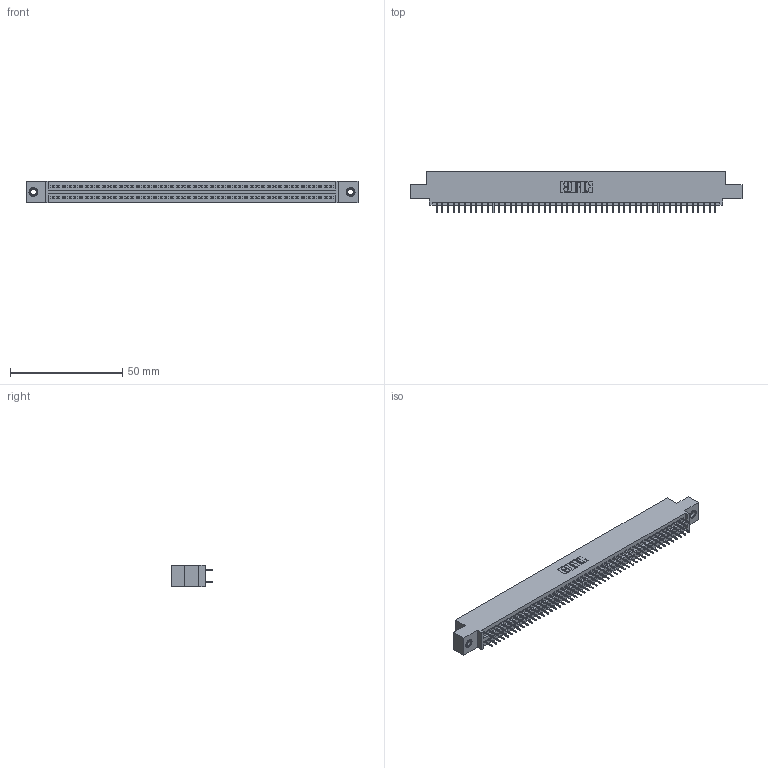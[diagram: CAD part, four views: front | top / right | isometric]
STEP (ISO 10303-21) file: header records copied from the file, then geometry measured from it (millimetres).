
FILE_DESCRIPTION (( 'STEP AP203' ), '1' );
FILE_NAME ('345-100-525-507.STEP', '2020-09-21T18:11:21', ( '' ), ( '' ), 'SwSTEP 2.0', 'SolidWorks 2020', '' );
FILE_SCHEMA (( 'CONFIG_CONTROL_DESIGN' ));
Length unit declared in the file: inch
Products named in the file (4): 345 Part_0.110 Offset - 0.156 Dia-TI; 345-100-525-507; 345-292-001_345-293-125; 345-250-001_345-250-005-103
Assembly tree (103 placements, depth 2):
  345-100-525-507
    345 Part_0.110 Offset - 0.156 Dia-TI
    345-292-001_345-293-125  x100
    345-250-001_345-250-005-103  x2
Bounding box: 148.21 x 18.72 x 9.4 mm (x, y, z)
Volume: 14219.9 mm3; surface area: 20799.1 mm2
Topology: 103 solids, 103 shells, 5590 faces, 15789 edges, 10118 vertices
Faces by surface type: plane 4016, cylinder 1558, cone 12, torus 4
Entity records: 39546 total; most frequent: CARTESIAN_POINT 6603, ORIENTED_EDGE 6530, DIRECTION 5839, EDGE_CURVE 3265, VECTOR 2917, LINE 2917, VERTEX_POINT 2168, AXIS2_PLACEMENT_3D 1461
